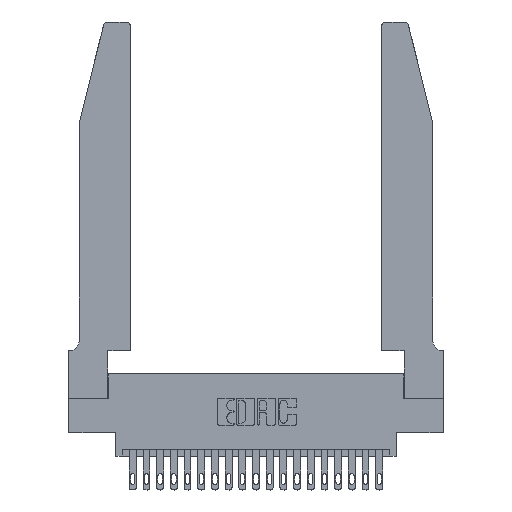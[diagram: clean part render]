
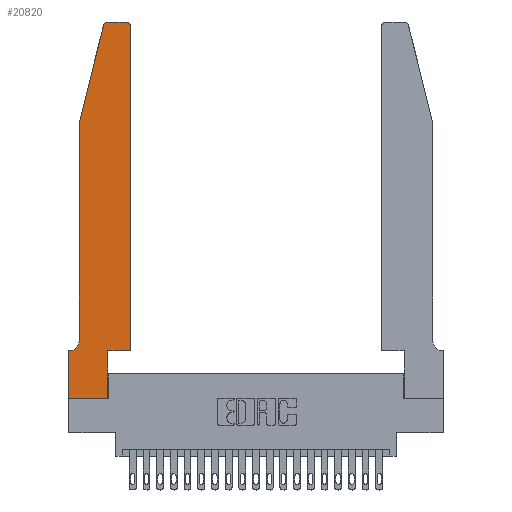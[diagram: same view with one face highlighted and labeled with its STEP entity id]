
A CAD part, top view. The second image highlights one B-rep face of the part: STEP entity #20820.
In plain terms, the highlighted planar face has unit normal (0, 0, 1).
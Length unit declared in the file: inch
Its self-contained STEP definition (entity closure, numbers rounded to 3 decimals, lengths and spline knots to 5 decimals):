
#315 = CARTESIAN_POINT ( 'NONE',  ( 0.0755, 0.35, 0.37 ) ) ;
#494 = CARTESIAN_POINT ( 'NONE',  ( 0.4205, 2.72, 0.37 ) ) ;
#620 = VERTEX_POINT ( 'NONE', #5432 ) ;
#1130 = ORIENTED_EDGE ( 'NONE', *, *, #19627, .T. ) ;
#1224 = CARTESIAN_POINT ( 'NONE',  ( 0.0755, 2., 0.37 ) ) ;
#1685 = VERTEX_POINT ( 'NONE', #4150 ) ;
#1810 = CIRCLE ( 'NONE', #15130, 0.03 ) ;
#2102 = CARTESIAN_POINT ( 'NONE',  ( 0.4505, 0.35, 0.37 ) ) ;
#2159 = LINE ( 'NONE', #14914, #11840 ) ;
#2286 = EDGE_CURVE ( 'NONE', #7706, #9724, #4139, .T. ) ;
#2383 = EDGE_CURVE ( 'NONE', #14455, #7525, #16817, .T. ) ;
#2515 = CARTESIAN_POINT ( 'NONE',  ( 0.4505, 0.35, 0.37 ) ) ;
#2671 = DIRECTION ( 'NONE',  ( 0., 1., 0. ) ) ;
#3081 = VECTOR ( 'NONE', #15298, 39.37008 ) ;
#3106 = DIRECTION ( 'NONE',  ( -1., 0., 0. ) ) ;
#3160 = VECTOR ( 'NONE', #3106, 39.37008 ) ;
#3714 = VECTOR ( 'NONE', #2671, 39.37008 ) ;
#3949 = DIRECTION ( 'NONE',  ( -0.239, -0.971, 0. ) ) ;
#4064 = EDGE_CURVE ( 'NONE', #620, #7114, #19758, .T. ) ;
#4139 = CIRCLE ( 'NONE', #12258, 0.07 ) ;
#4150 = CARTESIAN_POINT ( 'NONE',  ( 0.284, 2.75, 0.37 ) ) ;
#4268 = LINE ( 'NONE', #18445, #3714 ) ;
#4820 = VECTOR ( 'NONE', #21932, 39.37008 ) ;
#5222 = EDGE_CURVE ( 'NONE', #1685, #22674, #1810, .T. ) ;
#5432 = CARTESIAN_POINT ( 'NONE',  ( 0., 0.35, 0.37 ) ) ;
#5591 = EDGE_LOOP ( 'NONE', ( #5745, #6432, #18966, #18536, #6670, #7640, #21972, #22565, #1130, #16802, #11699, #21993 ) ) ;
#5729 = DIRECTION ( 'NONE',  ( -1., 0., 0. ) ) ;
#5745 = ORIENTED_EDGE ( 'NONE', *, *, #14254, .T. ) ;
#5836 = DIRECTION ( 'NONE',  ( 0., 0., 1. ) ) ;
#6099 = EDGE_CURVE ( 'NONE', #12669, #7706, #8137, .T. ) ;
#6432 = ORIENTED_EDGE ( 'NONE', *, *, #5222, .T. ) ;
#6661 = EDGE_CURVE ( 'NONE', #7114, #11147, #7775, .T. ) ;
#6670 = ORIENTED_EDGE ( 'NONE', *, *, #2286, .T. ) ;
#7114 = VERTEX_POINT ( 'NONE', #18556 ) ;
#7477 = LINE ( 'NONE', #315, #9137 ) ;
#7525 = VERTEX_POINT ( 'NONE', #20649 ) ;
#7640 = ORIENTED_EDGE ( 'NONE', *, *, #15849, .T. ) ;
#7706 = VERTEX_POINT ( 'NONE', #16718 ) ;
#7775 = LINE ( 'NONE', #15151, #3081 ) ;
#8046 = CARTESIAN_POINT ( 'NONE',  ( 0., 0.35, 0.37 ) ) ;
#8137 = LINE ( 'NONE', #22309, #9813 ) ;
#8308 = VERTEX_POINT ( 'NONE', #2102 ) ;
#8629 = EDGE_CURVE ( 'NONE', #22674, #12669, #2159, .T. ) ;
#9010 = CARTESIAN_POINT ( 'NONE',  ( 0.2865, 0.35, 0.37 ) ) ;
#9052 = DIRECTION ( 'NONE',  ( 0., -1., 0. ) ) ;
#9137 = VECTOR ( 'NONE', #9297, 39.37008 ) ;
#9297 = DIRECTION ( 'NONE',  ( -1., 0., 0. ) ) ;
#9724 = VERTEX_POINT ( 'NONE', #19464 ) ;
#9813 = VECTOR ( 'NONE', #18591, 39.37008 ) ;
#10073 = CARTESIAN_POINT ( 'NONE',  ( 0.2605, 2.75, 0.37 ) ) ;
#10114 = LINE ( 'NONE', #2515, #4820 ) ;
#10893 = LINE ( 'NONE', #10073, #3160 ) ;
#11147 = VERTEX_POINT ( 'NONE', #18317 ) ;
#11674 = DIRECTION ( 'NONE',  ( 0., 0., 1. ) ) ;
#11699 = ORIENTED_EDGE ( 'NONE', *, *, #19274, .T. ) ;
#11840 = VECTOR ( 'NONE', #3949, 39.37008 ) ;
#12258 = AXIS2_PLACEMENT_3D ( 'NONE', #12733, #15984, #5729 ) ;
#12622 = DIRECTION ( 'NONE',  ( 0., 1., 0. ) ) ;
#12669 = VERTEX_POINT ( 'NONE', #1224 ) ;
#12733 = CARTESIAN_POINT ( 'NONE',  ( 0.0055, 0.42, 0.37 ) ) ;
#12810 = DIRECTION ( 'NONE',  ( 0., 0., 1. ) ) ;
#13265 = EDGE_CURVE ( 'NONE', #17786, #8308, #10114, .T. ) ;
#14254 = EDGE_CURVE ( 'NONE', #7525, #1685, #10893, .T. ) ;
#14455 = VERTEX_POINT ( 'NONE', #19459 ) ;
#14914 = CARTESIAN_POINT ( 'NONE',  ( 0.0755, 2., 0.37 ) ) ;
#15130 = AXIS2_PLACEMENT_3D ( 'NONE', #20976, #5836, #18038 ) ;
#15151 = CARTESIAN_POINT ( 'NONE',  ( 0., 0., 0.37 ) ) ;
#15298 = DIRECTION ( 'NONE',  ( 1., 0., 0. ) ) ;
#15849 = EDGE_CURVE ( 'NONE', #9724, #620, #7477, .T. ) ;
#15984 = DIRECTION ( 'NONE',  ( 0., 0., -1. ) ) ;
#16718 = CARTESIAN_POINT ( 'NONE',  ( 0.0755, 0.42, 0.37 ) ) ;
#16782 = PLANE ( 'NONE',  #20486 ) ;
#16802 = ORIENTED_EDGE ( 'NONE', *, *, #13265, .T. ) ;
#16817 = CIRCLE ( 'NONE', #20207, 0.03 ) ;
#17786 = VERTEX_POINT ( 'NONE', #9010 ) ;
#18038 = DIRECTION ( 'NONE',  ( 1., 0., 0. ) ) ;
#18085 = DIRECTION ( 'NONE',  ( 1., 0., 0. ) ) ;
#18317 = CARTESIAN_POINT ( 'NONE',  ( 0.2865, 0., 0.37 ) ) ;
#18445 = CARTESIAN_POINT ( 'NONE',  ( 0.2865, 0.35, 0.37 ) ) ;
#18536 = ORIENTED_EDGE ( 'NONE', *, *, #6099, .T. ) ;
#18556 = CARTESIAN_POINT ( 'NONE',  ( 0., 0., 0.37 ) ) ;
#18591 = DIRECTION ( 'NONE',  ( 0., -1., 0. ) ) ;
#18700 = CARTESIAN_POINT ( 'NONE',  ( 0.25487, 2.72718, 0.37 ) ) ;
#18860 = LINE ( 'NONE', #19608, #21343 ) ;
#18930 = VECTOR ( 'NONE', #9052, 39.37008 ) ;
#18966 = ORIENTED_EDGE ( 'NONE', *, *, #8629, .T. ) ;
#19011 = FACE_OUTER_BOUND ( 'NONE', #5591, .T. ) ;
#19274 = EDGE_CURVE ( 'NONE', #8308, #14455, #18860, .T. ) ;
#19459 = CARTESIAN_POINT ( 'NONE',  ( 0.4505, 2.72, 0.37 ) ) ;
#19464 = CARTESIAN_POINT ( 'NONE',  ( 0.0055, 0.35, 0.37 ) ) ;
#19608 = CARTESIAN_POINT ( 'NONE',  ( 0.4505, 0.35, 0.37 ) ) ;
#19627 = EDGE_CURVE ( 'NONE', #11147, #17786, #4268, .T. ) ;
#19758 = LINE ( 'NONE', #21943, #18930 ) ;
#20207 = AXIS2_PLACEMENT_3D ( 'NONE', #494, #12810, #18085 ) ;
#20408 = DIRECTION ( 'NONE',  ( 1., 0., 0. ) ) ;
#20486 = AXIS2_PLACEMENT_3D ( 'NONE', #8046, #11674, #20408 ) ;
#20649 = CARTESIAN_POINT ( 'NONE',  ( 0.4205, 2.75, 0.37 ) ) ;
#20820 = ADVANCED_FACE ( 'NONE', ( #19011 ), #16782, .T. ) ;
#20976 = CARTESIAN_POINT ( 'NONE',  ( 0.284, 2.72, 0.37 ) ) ;
#21343 = VECTOR ( 'NONE', #12622, 39.37008 ) ;
#21932 = DIRECTION ( 'NONE',  ( 1., 0., 0. ) ) ;
#21943 = CARTESIAN_POINT ( 'NONE',  ( 0., 0., 0.37 ) ) ;
#21972 = ORIENTED_EDGE ( 'NONE', *, *, #4064, .T. ) ;
#21993 = ORIENTED_EDGE ( 'NONE', *, *, #2383, .T. ) ;
#22309 = CARTESIAN_POINT ( 'NONE',  ( 0.0755, 2., 0.37 ) ) ;
#22565 = ORIENTED_EDGE ( 'NONE', *, *, #6661, .T. ) ;
#22674 = VERTEX_POINT ( 'NONE', #18700 ) ;
